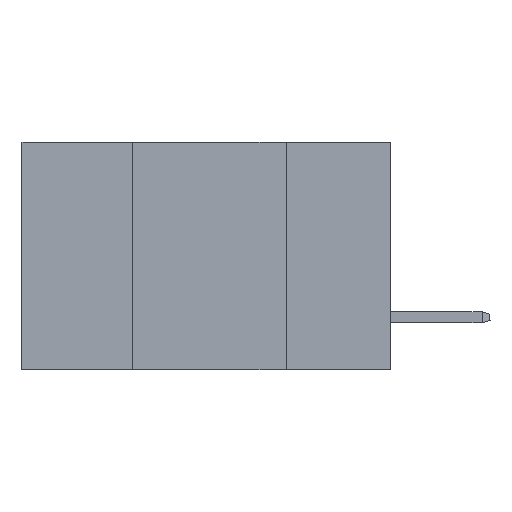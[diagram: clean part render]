
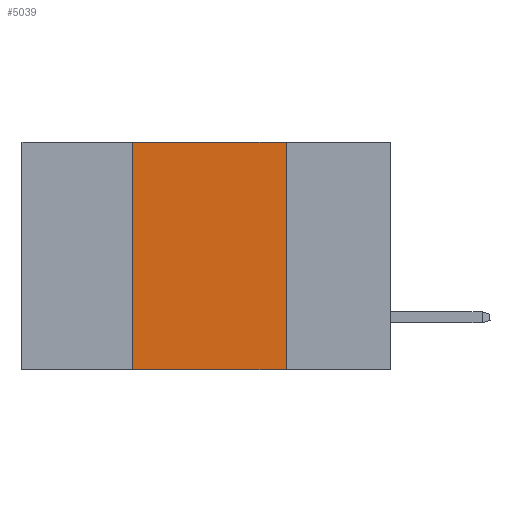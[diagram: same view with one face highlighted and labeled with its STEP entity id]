
A CAD part, left-side view. The second image highlights one B-rep face of the part: STEP entity #5039.
In plain terms, the highlighted planar face has unit normal (-1, 0, 0).
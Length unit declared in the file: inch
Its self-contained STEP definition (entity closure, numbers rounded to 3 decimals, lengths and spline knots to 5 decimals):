
#51 = EDGE_CURVE ( 'NONE', #13390, #20462, #16219, .T. ) ;
#77 = DIRECTION ( 'NONE',  ( 0., 0., 1. ) ) ;
#103 = ORIENTED_EDGE ( 'NONE', *, *, #18867, .F. ) ;
#258 = LINE ( 'NONE', #21119, #4048 ) ;
#348 = FACE_OUTER_BOUND ( 'NONE', #4112, .T. ) ;
#1108 = AXIS2_PLACEMENT_3D ( 'NONE', #1955, #21634, #15546 ) ;
#1343 = CARTESIAN_POINT ( 'NONE',  ( 0., 0.17, -0.37 ) ) ;
#1664 = DIRECTION ( 'NONE',  ( 0., 0., -1. ) ) ;
#1955 = CARTESIAN_POINT ( 'NONE',  ( 0., 0.6, 0. ) ) ;
#2418 = CARTESIAN_POINT ( 'NONE',  ( 0., 0.42, 0. ) ) ;
#4048 = VECTOR ( 'NONE', #18899, 39.37008 ) ;
#4112 = EDGE_LOOP ( 'NONE', ( #4890, #12850, #103, #25478 ) ) ;
#4254 = CARTESIAN_POINT ( 'NONE',  ( 0., 0.17, 0. ) ) ;
#4890 = ORIENTED_EDGE ( 'NONE', *, *, #51, .F. ) ;
#5039 = ADVANCED_FACE ( 'NONE', ( #348 ), #7185, .F. ) ;
#5494 = LINE ( 'NONE', #14777, #21565 ) ;
#7181 = CARTESIAN_POINT ( 'NONE',  ( 0., 0.42, -0.37 ) ) ;
#7185 = PLANE ( 'NONE',  #1108 ) ;
#10924 = VECTOR ( 'NONE', #1664, 39.37008 ) ;
#11121 = VECTOR ( 'NONE', #77, 39.37008 ) ;
#12850 = ORIENTED_EDGE ( 'NONE', *, *, #13395, .F. ) ;
#13390 = VERTEX_POINT ( 'NONE', #4254 ) ;
#13395 = EDGE_CURVE ( 'NONE', #23401, #13390, #5494, .T. ) ;
#13911 = CARTESIAN_POINT ( 'NONE',  ( 0., 0.42, 0. ) ) ;
#14777 = CARTESIAN_POINT ( 'NONE',  ( 0., 0.6, 0. ) ) ;
#15546 = DIRECTION ( 'NONE',  ( 0., 0., -1. ) ) ;
#16219 = LINE ( 'NONE', #25367, #10924 ) ;
#17069 = EDGE_CURVE ( 'NONE', #18329, #20462, #258, .T. ) ;
#18329 = VERTEX_POINT ( 'NONE', #7181 ) ;
#18867 = EDGE_CURVE ( 'NONE', #18329, #23401, #22854, .T. ) ;
#18899 = DIRECTION ( 'NONE',  ( 0., -1., 0. ) ) ;
#20462 = VERTEX_POINT ( 'NONE', #1343 ) ;
#21119 = CARTESIAN_POINT ( 'NONE',  ( 0., 0.6, -0.37 ) ) ;
#21565 = VECTOR ( 'NONE', #24258, 39.37008 ) ;
#21634 = DIRECTION ( 'NONE',  ( 1., 0., 0. ) ) ;
#22854 = LINE ( 'NONE', #13911, #11121 ) ;
#23401 = VERTEX_POINT ( 'NONE', #2418 ) ;
#24258 = DIRECTION ( 'NONE',  ( 0., -1., 0. ) ) ;
#25367 = CARTESIAN_POINT ( 'NONE',  ( 0., 0.17, 0. ) ) ;
#25478 = ORIENTED_EDGE ( 'NONE', *, *, #17069, .T. ) ;
